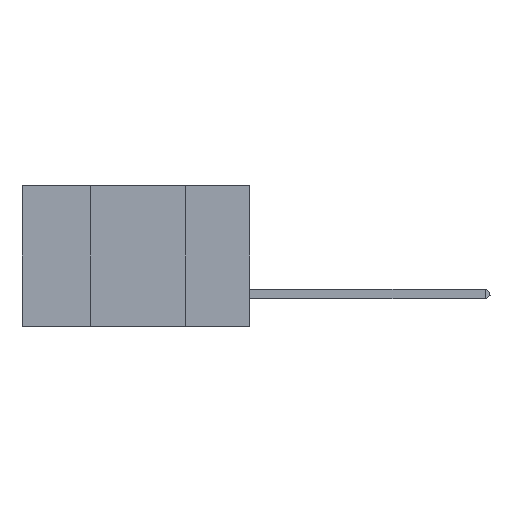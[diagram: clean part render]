
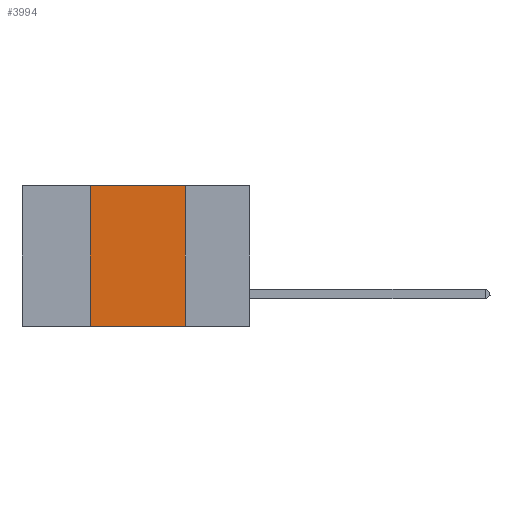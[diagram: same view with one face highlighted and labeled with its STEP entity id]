
A CAD part, left-side view. The second image highlights one B-rep face of the part: STEP entity #3994.
In plain terms, the highlighted planar face has unit normal (-1, 0, 0).
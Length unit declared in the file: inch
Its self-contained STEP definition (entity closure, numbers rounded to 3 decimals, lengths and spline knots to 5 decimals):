
#504 = VECTOR ( 'NONE', #19948, 39.37008 ) ;
#836 = CARTESIAN_POINT ( 'NONE',  ( 0., 0.6, 0. ) ) ;
#1516 = CARTESIAN_POINT ( 'NONE',  ( 0., 0.17, 0. ) ) ;
#1757 = EDGE_CURVE ( 'NONE', #12043, #16777, #2318, .T. ) ;
#1819 = VECTOR ( 'NONE', #17467, 39.37008 ) ;
#1909 = AXIS2_PLACEMENT_3D ( 'NONE', #7037, #14797, #8625 ) ;
#2012 = DIRECTION ( 'NONE',  ( 0., 0., -1. ) ) ;
#2291 = VERTEX_POINT ( 'NONE', #6475 ) ;
#2318 = LINE ( 'NONE', #6812, #19001 ) ;
#2927 = ORIENTED_EDGE ( 'NONE', *, *, #1757, .F. ) ;
#3109 = CARTESIAN_POINT ( 'NONE',  ( 0., 0.42, 0. ) ) ;
#3387 = CARTESIAN_POINT ( 'NONE',  ( 0., 0.6, -0.37 ) ) ;
#3482 = LINE ( 'NONE', #836, #504 ) ;
#3994 = ADVANCED_FACE ( 'NONE', ( #9917 ), #17963, .F. ) ;
#4137 = ORIENTED_EDGE ( 'NONE', *, *, #12076, .T. ) ;
#6475 = CARTESIAN_POINT ( 'NONE',  ( 0., 0.42, -0.37 ) ) ;
#6812 = CARTESIAN_POINT ( 'NONE',  ( 0., 0.17, 0. ) ) ;
#7037 = CARTESIAN_POINT ( 'NONE',  ( 0., 0.6, 0. ) ) ;
#8537 = VERTEX_POINT ( 'NONE', #9870 ) ;
#8625 = DIRECTION ( 'NONE',  ( 0., 0., -1. ) ) ;
#9451 = ORIENTED_EDGE ( 'NONE', *, *, #11488, .F. ) ;
#9469 = EDGE_CURVE ( 'NONE', #2291, #8537, #13526, .T. ) ;
#9870 = CARTESIAN_POINT ( 'NONE',  ( 0., 0.42, 0. ) ) ;
#9917 = FACE_OUTER_BOUND ( 'NONE', #13981, .T. ) ;
#11488 = EDGE_CURVE ( 'NONE', #8537, #12043, #3482, .T. ) ;
#12043 = VERTEX_POINT ( 'NONE', #1516 ) ;
#12076 = EDGE_CURVE ( 'NONE', #2291, #16777, #12377, .T. ) ;
#12377 = LINE ( 'NONE', #3387, #15637 ) ;
#13526 = LINE ( 'NONE', #3109, #1819 ) ;
#13981 = EDGE_LOOP ( 'NONE', ( #2927, #9451, #14388, #4137 ) ) ;
#14224 = DIRECTION ( 'NONE',  ( 0., -1., 0. ) ) ;
#14388 = ORIENTED_EDGE ( 'NONE', *, *, #9469, .F. ) ;
#14797 = DIRECTION ( 'NONE',  ( 1., 0., 0. ) ) ;
#15637 = VECTOR ( 'NONE', #14224, 39.37008 ) ;
#16777 = VERTEX_POINT ( 'NONE', #18410 ) ;
#17467 = DIRECTION ( 'NONE',  ( 0., 0., 1. ) ) ;
#17963 = PLANE ( 'NONE',  #1909 ) ;
#18410 = CARTESIAN_POINT ( 'NONE',  ( 0., 0.17, -0.37 ) ) ;
#19001 = VECTOR ( 'NONE', #2012, 39.37008 ) ;
#19948 = DIRECTION ( 'NONE',  ( 0., -1., 0. ) ) ;
